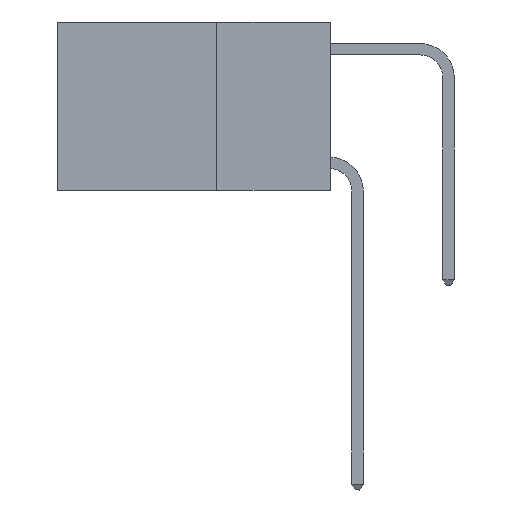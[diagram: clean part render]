
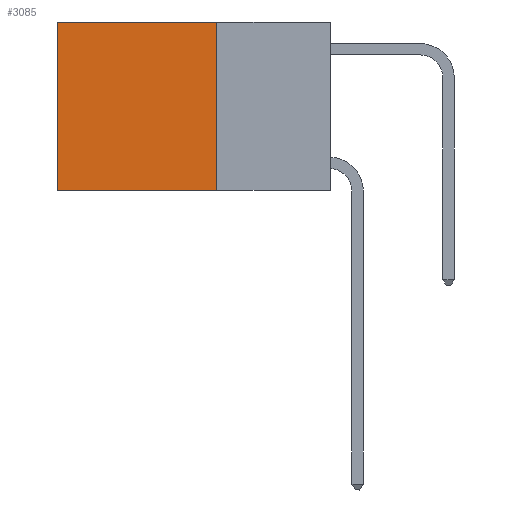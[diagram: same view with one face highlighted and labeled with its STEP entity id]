
A CAD part, left-side view. The second image highlights one B-rep face of the part: STEP entity #3085.
In plain terms, the highlighted planar face has unit normal (-1, 0, 0).
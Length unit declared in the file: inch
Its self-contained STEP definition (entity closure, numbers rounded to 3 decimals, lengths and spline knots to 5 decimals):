
#887 = FACE_OUTER_BOUND ( 'NONE', #5454, .T. ) ;
#1771 = VECTOR ( 'NONE', #11181, 39.37008 ) ;
#2515 = CARTESIAN_POINT ( 'NONE',  ( 0.2625, 0.6, 0. ) ) ;
#2847 = LINE ( 'NONE', #9453, #11460 ) ;
#3085 = ADVANCED_FACE ( 'NONE', ( #887 ), #13991, .F. ) ;
#3778 = ORIENTED_EDGE ( 'NONE', *, *, #17450, .T. ) ;
#4092 = ORIENTED_EDGE ( 'NONE', *, *, #9290, .F. ) ;
#4734 = AXIS2_PLACEMENT_3D ( 'NONE', #15640, #17217, #7475 ) ;
#4899 = DIRECTION ( 'NONE',  ( 0., 1., 0. ) ) ;
#5454 = EDGE_LOOP ( 'NONE', ( #3778, #4092, #5510, #13145 ) ) ;
#5510 = ORIENTED_EDGE ( 'NONE', *, *, #20012, .F. ) ;
#5623 = CARTESIAN_POINT ( 'NONE',  ( 0.2625, 0.6, -0.37 ) ) ;
#6091 = DIRECTION ( 'NONE',  ( 0., 1., 0. ) ) ;
#6258 = VERTEX_POINT ( 'NONE', #5623 ) ;
#6539 = CARTESIAN_POINT ( 'NONE',  ( 0.2625, 0.25, 0. ) ) ;
#7475 = DIRECTION ( 'NONE',  ( 0., 0., -1. ) ) ;
#7803 = CARTESIAN_POINT ( 'NONE',  ( 0.2625, 0.25, -0.37 ) ) ;
#9290 = EDGE_CURVE ( 'NONE', #9787, #6258, #17168, .T. ) ;
#9453 = CARTESIAN_POINT ( 'NONE',  ( 0.2625, 0.25, 0. ) ) ;
#9787 = VERTEX_POINT ( 'NONE', #7803 ) ;
#10940 = LINE ( 'NONE', #2515, #1771 ) ;
#11181 = DIRECTION ( 'NONE',  ( 0., 0., -1. ) ) ;
#11460 = VECTOR ( 'NONE', #6091, 39.37008 ) ;
#12289 = CARTESIAN_POINT ( 'NONE',  ( 0.2625, 0.6, 0. ) ) ;
#12977 = CARTESIAN_POINT ( 'NONE',  ( 0.2625, 0.25, 0. ) ) ;
#13145 = ORIENTED_EDGE ( 'NONE', *, *, #17397, .T. ) ;
#13344 = VERTEX_POINT ( 'NONE', #12977 ) ;
#13991 = PLANE ( 'NONE',  #4734 ) ;
#14741 = DIRECTION ( 'NONE',  ( 0., 0., -1. ) ) ;
#15640 = CARTESIAN_POINT ( 'NONE',  ( 0.2625, 0.25, 0. ) ) ;
#16267 = VERTEX_POINT ( 'NONE', #12289 ) ;
#17168 = LINE ( 'NONE', #18093, #17669 ) ;
#17193 = LINE ( 'NONE', #6539, #19877 ) ;
#17217 = DIRECTION ( 'NONE',  ( 1., 0., 0. ) ) ;
#17397 = EDGE_CURVE ( 'NONE', #13344, #16267, #2847, .T. ) ;
#17450 = EDGE_CURVE ( 'NONE', #16267, #6258, #10940, .T. ) ;
#17669 = VECTOR ( 'NONE', #4899, 39.37008 ) ;
#18093 = CARTESIAN_POINT ( 'NONE',  ( 0.2625, 0.25, -0.37 ) ) ;
#19877 = VECTOR ( 'NONE', #14741, 39.37008 ) ;
#20012 = EDGE_CURVE ( 'NONE', #13344, #9787, #17193, .T. ) ;
